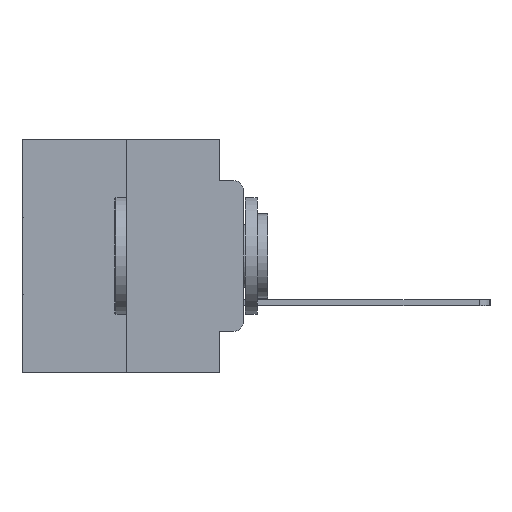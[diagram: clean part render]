
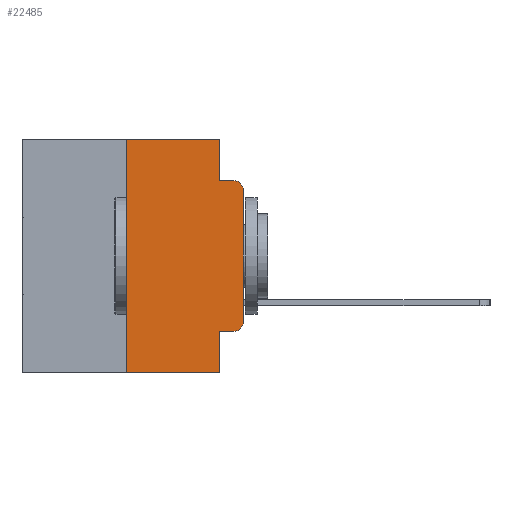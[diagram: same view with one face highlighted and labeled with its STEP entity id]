
A CAD part, left-side view. The second image highlights one B-rep face of the part: STEP entity #22485.
In plain terms, the highlighted planar face has unit normal (-1, 0, 0).
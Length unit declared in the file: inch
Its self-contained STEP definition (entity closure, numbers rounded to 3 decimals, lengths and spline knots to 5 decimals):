
#145 = VERTEX_POINT ( 'NONE', #8441 ) ;
#493 = DIRECTION ( 'NONE',  ( 0., -1., 0. ) ) ;
#538 = LINE ( 'NONE', #28109, #13279 ) ;
#1276 = DIRECTION ( 'NONE',  ( -1., 0., 0. ) ) ;
#1848 = DIRECTION ( 'NONE',  ( 1., 0., 0. ) ) ;
#2484 = EDGE_CURVE ( 'NONE', #6576, #145, #28027, .T. ) ;
#3454 = CARTESIAN_POINT ( 'NONE',  ( 0., 0.02, -0.3915 ) ) ;
#3586 = ORIENTED_EDGE ( 'NONE', *, *, #14124, .T. ) ;
#3947 = ORIENTED_EDGE ( 'NONE', *, *, #21425, .F. ) ;
#4317 = CARTESIAN_POINT ( 'NONE',  ( 0., 0.25, 0. ) ) ;
#4444 = VERTEX_POINT ( 'NONE', #26160 ) ;
#4614 = VECTOR ( 'NONE', #13575, 39.37008 ) ;
#4681 = ORIENTED_EDGE ( 'NONE', *, *, #23366, .F. ) ;
#4706 = EDGE_CURVE ( 'NONE', #12568, #21041, #20605, .T. ) ;
#4950 = VECTOR ( 'NONE', #28623, 39.37008 ) ;
#4982 = EDGE_CURVE ( 'NONE', #5474, #17337, #538, .T. ) ;
#5474 = VERTEX_POINT ( 'NONE', #23347 ) ;
#5846 = DIRECTION ( 'NONE',  ( 0., 0., -1. ) ) ;
#6576 = VERTEX_POINT ( 'NONE', #15857 ) ;
#6584 = CARTESIAN_POINT ( 'NONE',  ( 0., 0.473, 0. ) ) ;
#7269 = CARTESIAN_POINT ( 'NONE',  ( 0., 0.051, -0.5 ) ) ;
#7589 = CARTESIAN_POINT ( 'NONE',  ( 0., 0.25, 0. ) ) ;
#8037 = ORIENTED_EDGE ( 'NONE', *, *, #30257, .T. ) ;
#8441 = CARTESIAN_POINT ( 'NONE',  ( 0., 0.02, -0.4115 ) ) ;
#8546 = VERTEX_POINT ( 'NONE', #13968 ) ;
#9386 = VECTOR ( 'NONE', #493, 39.37008 ) ;
#10463 = CARTESIAN_POINT ( 'NONE',  ( 0., 0.051, -0.4115 ) ) ;
#10933 = CARTESIAN_POINT ( 'NONE',  ( 0., 0., -0.1085 ) ) ;
#11183 = CARTESIAN_POINT ( 'NONE',  ( 0., 0.473, -0.5 ) ) ;
#11417 = AXIS2_PLACEMENT_3D ( 'NONE', #15547, #1276, #17903 ) ;
#11945 = LINE ( 'NONE', #13239, #29734 ) ;
#12045 = CIRCLE ( 'NONE', #23287, 0.02 ) ;
#12106 = AXIS2_PLACEMENT_3D ( 'NONE', #23028, #1848, #18451 ) ;
#12315 = CARTESIAN_POINT ( 'NONE',  ( 0., 0.02, -0.0885 ) ) ;
#12568 = VERTEX_POINT ( 'NONE', #10933 ) ;
#13224 = EDGE_CURVE ( 'NONE', #4444, #26741, #23386, .T. ) ;
#13239 = CARTESIAN_POINT ( 'NONE',  ( 0., 0.051, -0.0885 ) ) ;
#13279 = VECTOR ( 'NONE', #16547, 39.37008 ) ;
#13575 = DIRECTION ( 'NONE',  ( 0., -1., 0. ) ) ;
#13968 = CARTESIAN_POINT ( 'NONE',  ( 0., 0., -0.3915 ) ) ;
#14124 = EDGE_CURVE ( 'NONE', #145, #8546, #12045, .T. ) ;
#14326 = ORIENTED_EDGE ( 'NONE', *, *, #4706, .T. ) ;
#14619 = EDGE_CURVE ( 'NONE', #6576, #26741, #23728, .T. ) ;
#14871 = EDGE_LOOP ( 'NONE', ( #8037, #14326, #15812, #28143, #3947, #4681, #19460, #27106, #15458, #3586 ) ) ;
#15084 = VECTOR ( 'NONE', #18440, 39.37008 ) ;
#15458 = ORIENTED_EDGE ( 'NONE', *, *, #2484, .T. ) ;
#15470 = EDGE_CURVE ( 'NONE', #17337, #21041, #11945, .T. ) ;
#15547 = CARTESIAN_POINT ( 'NONE',  ( 0., 0.02, -0.1085 ) ) ;
#15736 = FACE_OUTER_BOUND ( 'NONE', #14871, .T. ) ;
#15812 = ORIENTED_EDGE ( 'NONE', *, *, #15470, .F. ) ;
#15857 = CARTESIAN_POINT ( 'NONE',  ( 0., 0.051, -0.4115 ) ) ;
#15920 = DIRECTION ( 'NONE',  ( 0., 0., 1. ) ) ;
#16547 = DIRECTION ( 'NONE',  ( 0., 0., -1. ) ) ;
#16721 = CARTESIAN_POINT ( 'NONE',  ( 0., 0.051, -0.0885 ) ) ;
#16980 = DIRECTION ( 'NONE',  ( 0., 0., 1. ) ) ;
#17337 = VERTEX_POINT ( 'NONE', #16721 ) ;
#17903 = DIRECTION ( 'NONE',  ( 0., 0., -1. ) ) ;
#18256 = CARTESIAN_POINT ( 'NONE',  ( 0., 0., 0. ) ) ;
#18440 = DIRECTION ( 'NONE',  ( 0., -1., 0. ) ) ;
#18451 = DIRECTION ( 'NONE',  ( 0., 0., -1. ) ) ;
#19460 = ORIENTED_EDGE ( 'NONE', *, *, #13224, .T. ) ;
#19968 = DIRECTION ( 'NONE',  ( -1., 0., 0. ) ) ;
#20605 = CIRCLE ( 'NONE', #11417, 0.02 ) ;
#21041 = VERTEX_POINT ( 'NONE', #12315 ) ;
#21295 = LINE ( 'NONE', #6584, #15084 ) ;
#21425 = EDGE_CURVE ( 'NONE', #30290, #5474, #21295, .T. ) ;
#21883 = VECTOR ( 'NONE', #16980, 39.37008 ) ;
#22485 = ADVANCED_FACE ( 'NONE', ( #15736 ), #29932, .F. ) ;
#23028 = CARTESIAN_POINT ( 'NONE',  ( 0., 0.473, 0. ) ) ;
#23287 = AXIS2_PLACEMENT_3D ( 'NONE', #3454, #19968, #5846 ) ;
#23347 = CARTESIAN_POINT ( 'NONE',  ( 0., 0.051, 0. ) ) ;
#23366 = EDGE_CURVE ( 'NONE', #4444, #30290, #28727, .T. ) ;
#23386 = LINE ( 'NONE', #11183, #4614 ) ;
#23728 = LINE ( 'NONE', #24022, #4950 ) ;
#23739 = VECTOR ( 'NONE', #15920, 39.37008 ) ;
#24022 = CARTESIAN_POINT ( 'NONE',  ( 0., 0.051, 0. ) ) ;
#26160 = CARTESIAN_POINT ( 'NONE',  ( 0., 0.25, -0.5 ) ) ;
#26741 = VERTEX_POINT ( 'NONE', #7269 ) ;
#27106 = ORIENTED_EDGE ( 'NONE', *, *, #14619, .F. ) ;
#28027 = LINE ( 'NONE', #10463, #9386 ) ;
#28109 = CARTESIAN_POINT ( 'NONE',  ( 0., 0.051, 0. ) ) ;
#28143 = ORIENTED_EDGE ( 'NONE', *, *, #4982, .F. ) ;
#28623 = DIRECTION ( 'NONE',  ( 0., 0., -1. ) ) ;
#28727 = LINE ( 'NONE', #7589, #21883 ) ;
#29456 = DIRECTION ( 'NONE',  ( 0., -1., 0. ) ) ;
#29734 = VECTOR ( 'NONE', #29456, 39.37008 ) ;
#29802 = LINE ( 'NONE', #18256, #23739 ) ;
#29932 = PLANE ( 'NONE',  #12106 ) ;
#30257 = EDGE_CURVE ( 'NONE', #8546, #12568, #29802, .T. ) ;
#30290 = VERTEX_POINT ( 'NONE', #4317 ) ;
